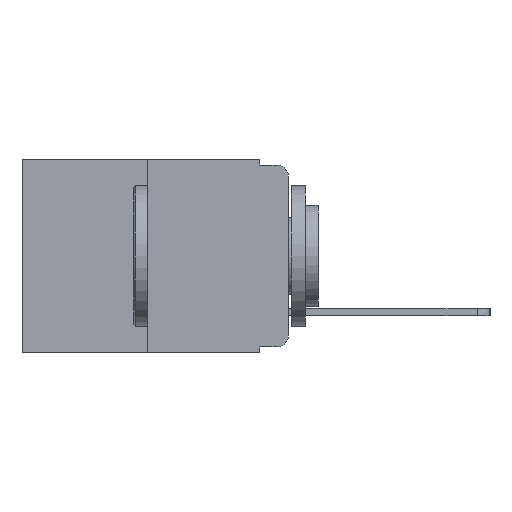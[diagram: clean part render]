
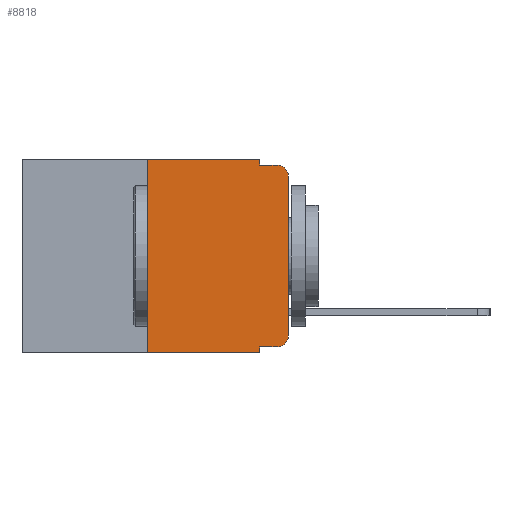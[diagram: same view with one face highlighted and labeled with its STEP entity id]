
A CAD part, left-side view. The second image highlights one B-rep face of the part: STEP entity #8818.
In plain terms, the highlighted planar face has unit normal (-1, 0, 0).
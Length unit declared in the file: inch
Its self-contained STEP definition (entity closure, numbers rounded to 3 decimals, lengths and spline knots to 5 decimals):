
#1281 = CARTESIAN_POINT ( 'NONE',  ( 0., 0.02, -0.01 ) ) ;
#1455 = CARTESIAN_POINT ( 'NONE',  ( 0., 0.051, -0.01 ) ) ;
#1508 = VECTOR ( 'NONE', #6670, 39.37008 ) ;
#1765 = VERTEX_POINT ( 'NONE', #13318 ) ;
#2072 = LINE ( 'NONE', #15562, #15064 ) ;
#2233 = EDGE_CURVE ( 'NONE', #6236, #6952, #17644, .T. ) ;
#2444 = VERTEX_POINT ( 'NONE', #9738 ) ;
#2974 = EDGE_CURVE ( 'NONE', #7853, #2444, #12309, .T. ) ;
#3581 = CARTESIAN_POINT ( 'NONE',  ( 0., 0.02, -0.313 ) ) ;
#3653 = VECTOR ( 'NONE', #7751, 39.37008 ) ;
#3784 = CIRCLE ( 'NONE', #20471, 0.02 ) ;
#3903 = CARTESIAN_POINT ( 'NONE',  ( 0., 0., -0.03 ) ) ;
#4048 = CARTESIAN_POINT ( 'NONE',  ( 0., 0.051, 0. ) ) ;
#4270 = CARTESIAN_POINT ( 'NONE',  ( 0., 0.051, -0.343 ) ) ;
#4318 = DIRECTION ( 'NONE',  ( 0., 0., 1. ) ) ;
#4604 = ORIENTED_EDGE ( 'NONE', *, *, #15196, .F. ) ;
#4936 = CIRCLE ( 'NONE', #17219, 0.02 ) ;
#4966 = ORIENTED_EDGE ( 'NONE', *, *, #16190, .T. ) ;
#5253 = DIRECTION ( 'NONE',  ( 0., 0., -1. ) ) ;
#5535 = VECTOR ( 'NONE', #7150, 39.37008 ) ;
#5537 = ORIENTED_EDGE ( 'NONE', *, *, #19160, .T. ) ;
#5622 = DIRECTION ( 'NONE',  ( -1., 0., 0. ) ) ;
#5666 = EDGE_CURVE ( 'NONE', #6236, #9665, #8585, .T. ) ;
#5914 = VERTEX_POINT ( 'NONE', #3903 ) ;
#6092 = CARTESIAN_POINT ( 'NONE',  ( 0., 0.25, 0. ) ) ;
#6150 = VECTOR ( 'NONE', #12131, 39.37008 ) ;
#6164 = VERTEX_POINT ( 'NONE', #9879 ) ;
#6236 = VERTEX_POINT ( 'NONE', #17868 ) ;
#6574 = DIRECTION ( 'NONE',  ( 0., 0., -1. ) ) ;
#6670 = DIRECTION ( 'NONE',  ( 0., -1., 0. ) ) ;
#6952 = VERTEX_POINT ( 'NONE', #13860 ) ;
#6954 = AXIS2_PLACEMENT_3D ( 'NONE', #8135, #16061, #6574 ) ;
#7132 = VERTEX_POINT ( 'NONE', #1281 ) ;
#7150 = DIRECTION ( 'NONE',  ( 0., -1., 0. ) ) ;
#7696 = FACE_OUTER_BOUND ( 'NONE', #12063, .T. ) ;
#7751 = DIRECTION ( 'NONE',  ( 0., 0., 1. ) ) ;
#7853 = VERTEX_POINT ( 'NONE', #15473 ) ;
#8135 = CARTESIAN_POINT ( 'NONE',  ( 0., 0.473, 0. ) ) ;
#8585 = LINE ( 'NONE', #9749, #16425 ) ;
#8818 = ADVANCED_FACE ( 'NONE', ( #7696 ), #14542, .F. ) ;
#9418 = LINE ( 'NONE', #11148, #17223 ) ;
#9559 = DIRECTION ( 'NONE',  ( 0., -1., 0. ) ) ;
#9665 = VERTEX_POINT ( 'NONE', #4270 ) ;
#9738 = CARTESIAN_POINT ( 'NONE',  ( 0., 0.25, 0. ) ) ;
#9749 = CARTESIAN_POINT ( 'NONE',  ( 0., 0.051, 0. ) ) ;
#9879 = CARTESIAN_POINT ( 'NONE',  ( 0., 0.051, -0.01 ) ) ;
#10318 = CARTESIAN_POINT ( 'NONE',  ( 0., 0.051, 0. ) ) ;
#10407 = ORIENTED_EDGE ( 'NONE', *, *, #19621, .T. ) ;
#10449 = ORIENTED_EDGE ( 'NONE', *, *, #2233, .T. ) ;
#10883 = EDGE_CURVE ( 'NONE', #7853, #9665, #9418, .T. ) ;
#11148 = CARTESIAN_POINT ( 'NONE',  ( 0., 0.473, -0.343 ) ) ;
#11152 = VECTOR ( 'NONE', #11375, 39.37008 ) ;
#11375 = DIRECTION ( 'NONE',  ( 0., -1., 0. ) ) ;
#11806 = EDGE_CURVE ( 'NONE', #2444, #16130, #13580, .T. ) ;
#12063 = EDGE_LOOP ( 'NONE', ( #5537, #4966, #4604, #14078, #19692, #19400, #17298, #17585, #10449, #10407 ) ) ;
#12131 = DIRECTION ( 'NONE',  ( 0., 0., -1. ) ) ;
#12309 = LINE ( 'NONE', #6092, #3653 ) ;
#13108 = CARTESIAN_POINT ( 'NONE',  ( 0., 0.051, -0.333 ) ) ;
#13318 = CARTESIAN_POINT ( 'NONE',  ( 0., 0., -0.313 ) ) ;
#13580 = LINE ( 'NONE', #16581, #5535 ) ;
#13860 = CARTESIAN_POINT ( 'NONE',  ( 0., 0.02, -0.333 ) ) ;
#14078 = ORIENTED_EDGE ( 'NONE', *, *, #14169, .F. ) ;
#14169 = EDGE_CURVE ( 'NONE', #16130, #6164, #18634, .T. ) ;
#14542 = PLANE ( 'NONE',  #6954 ) ;
#14880 = DIRECTION ( 'NONE',  ( -1., 0., 0. ) ) ;
#15064 = VECTOR ( 'NONE', #4318, 39.37008 ) ;
#15196 = EDGE_CURVE ( 'NONE', #6164, #7132, #15329, .T. ) ;
#15214 = CARTESIAN_POINT ( 'NONE',  ( 0., 0.02, -0.03 ) ) ;
#15329 = LINE ( 'NONE', #1455, #11152 ) ;
#15473 = CARTESIAN_POINT ( 'NONE',  ( 0., 0.25, -0.343 ) ) ;
#15562 = CARTESIAN_POINT ( 'NONE',  ( 0., 0., 0. ) ) ;
#15982 = DIRECTION ( 'NONE',  ( 0., 0., -1. ) ) ;
#16061 = DIRECTION ( 'NONE',  ( 1., 0., 0. ) ) ;
#16130 = VERTEX_POINT ( 'NONE', #10318 ) ;
#16190 = EDGE_CURVE ( 'NONE', #5914, #7132, #3784, .T. ) ;
#16425 = VECTOR ( 'NONE', #15982, 39.37008 ) ;
#16581 = CARTESIAN_POINT ( 'NONE',  ( 0., 0.473, 0. ) ) ;
#16694 = DIRECTION ( 'NONE',  ( 0., 0., -1. ) ) ;
#17219 = AXIS2_PLACEMENT_3D ( 'NONE', #3581, #14880, #5253 ) ;
#17223 = VECTOR ( 'NONE', #9559, 39.37008 ) ;
#17298 = ORIENTED_EDGE ( 'NONE', *, *, #10883, .T. ) ;
#17585 = ORIENTED_EDGE ( 'NONE', *, *, #5666, .F. ) ;
#17644 = LINE ( 'NONE', #13108, #1508 ) ;
#17868 = CARTESIAN_POINT ( 'NONE',  ( 0., 0.051, -0.333 ) ) ;
#18634 = LINE ( 'NONE', #4048, #6150 ) ;
#19160 = EDGE_CURVE ( 'NONE', #1765, #5914, #2072, .T. ) ;
#19400 = ORIENTED_EDGE ( 'NONE', *, *, #2974, .F. ) ;
#19621 = EDGE_CURVE ( 'NONE', #6952, #1765, #4936, .T. ) ;
#19692 = ORIENTED_EDGE ( 'NONE', *, *, #11806, .F. ) ;
#20471 = AXIS2_PLACEMENT_3D ( 'NONE', #15214, #5622, #16694 ) ;
